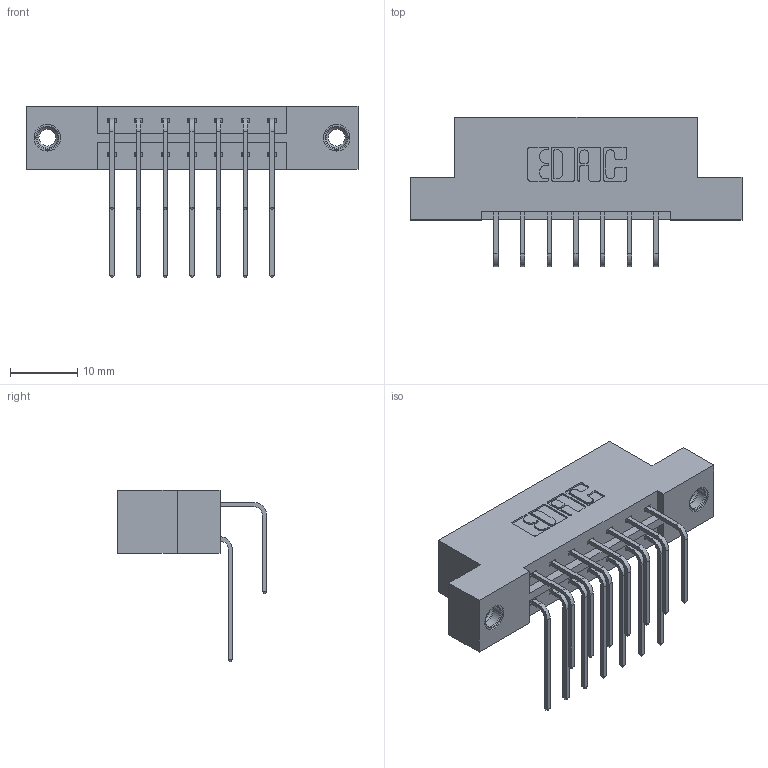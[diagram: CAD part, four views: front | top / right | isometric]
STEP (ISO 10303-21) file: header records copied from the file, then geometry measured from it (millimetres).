
FILE_DESCRIPTION (( 'STEP AP203' ), '1' );
FILE_NAME ('833-014-558-207.STEP', '2020-05-31T14:53:05', ( '' ), ( '' ), 'SwSTEP 2.0', 'SolidWorks 2020', '' );
FILE_SCHEMA (( 'CONFIG_CONTROL_DESIGN' ));
Length unit declared in the file: inch
Products named in the file (5): 345-292-001_558 559 Tail - 1; 345-250-001_345-250-005-103; 833-014-558-207; 345-292-001_558 Tail - 2; 833 Part_Flush - .156 Dia - TI
Assembly tree (17 placements, depth 2):
  833-014-558-207
    833 Part_Flush - .156 Dia - TI
    345-292-001_558 559 Tail - 1  x7
    345-292-001_558 Tail - 2  x7
    345-250-001_345-250-005-103  x2
Bounding box: 49.28 x 22.17 x 25.53 mm (x, y, z)
Volume: 4770.7 mm3; surface area: 5700.5 mm2
Topology: 17 solids, 17 shells, 930 faces, 2701 edges, 1774 vertices
Faces by surface type: plane 634, cylinder 280, cone 12, torus 4
Entity records: 12000 total; most frequent: CARTESIAN_POINT 2064, ORIENTED_EDGE 1942, DIRECTION 1837, EDGE_CURVE 971, VECTOR 783, LINE 783, VERTEX_POINT 640, AXIS2_PLACEMENT_3D 527
